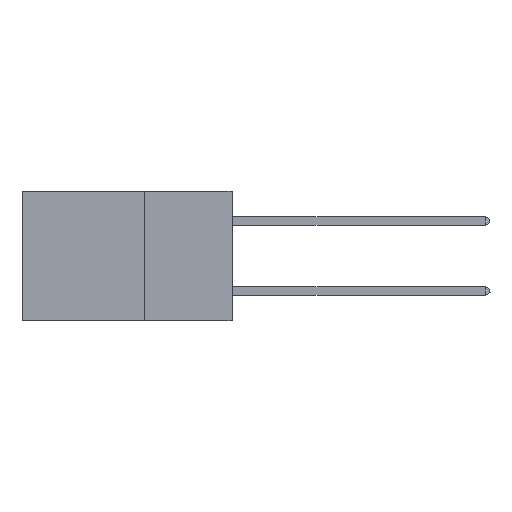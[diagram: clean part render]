
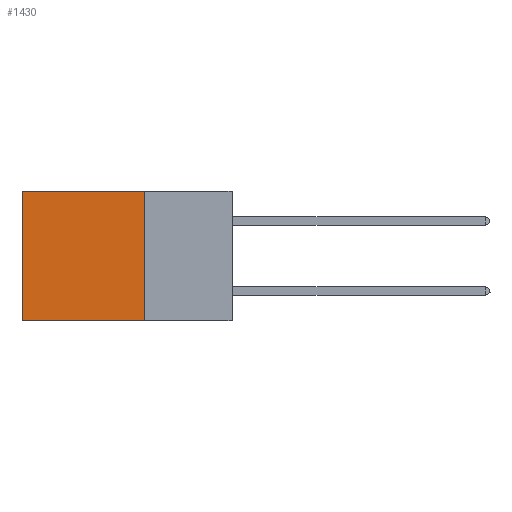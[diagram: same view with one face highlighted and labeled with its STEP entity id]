
A CAD part, left-side view. The second image highlights one B-rep face of the part: STEP entity #1430.
In plain terms, the highlighted planar face has unit normal (-1, 0, 0).
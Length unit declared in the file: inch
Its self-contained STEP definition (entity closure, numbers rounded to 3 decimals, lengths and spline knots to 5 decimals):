
#1430 = ADVANCED_FACE ( 'NONE', ( #26411 ), #11141, .F. ) ;
#1748 = VECTOR ( 'NONE', #10287, 39.37008 ) ;
#2034 = CARTESIAN_POINT ( 'NONE',  ( 0.2875, 0.25, 0. ) ) ;
#2132 = EDGE_CURVE ( 'NONE', #10776, #23455, #20278, .T. ) ;
#3590 = CARTESIAN_POINT ( 'NONE',  ( 0.2875, 0.25, -0.37 ) ) ;
#4003 = CARTESIAN_POINT ( 'NONE',  ( 0.2875, 0.6, -0.37 ) ) ;
#6883 = VERTEX_POINT ( 'NONE', #15807 ) ;
#7451 = CARTESIAN_POINT ( 'NONE',  ( 0.2875, 0.6, 0. ) ) ;
#9181 = LINE ( 'NONE', #15652, #20082 ) ;
#9241 = CARTESIAN_POINT ( 'NONE',  ( 0.2875, 0.25, 0. ) ) ;
#10201 = ORIENTED_EDGE ( 'NONE', *, *, #2132, .T. ) ;
#10287 = DIRECTION ( 'NONE',  ( 0., 1., 0. ) ) ;
#10776 = VERTEX_POINT ( 'NONE', #7451 ) ;
#11141 = PLANE ( 'NONE',  #11647 ) ;
#11647 = AXIS2_PLACEMENT_3D ( 'NONE', #9241, #23399, #19271 ) ;
#14461 = EDGE_CURVE ( 'NONE', #6883, #18330, #24735, .T. ) ;
#15525 = CARTESIAN_POINT ( 'NONE',  ( 0.2875, 0.25, -0.37 ) ) ;
#15572 = DIRECTION ( 'NONE',  ( 0., 1., 0. ) ) ;
#15652 = CARTESIAN_POINT ( 'NONE',  ( 0.2875, 0.25, 0. ) ) ;
#15807 = CARTESIAN_POINT ( 'NONE',  ( 0.2875, 0.25, 0. ) ) ;
#15849 = ORIENTED_EDGE ( 'NONE', *, *, #14461, .F. ) ;
#18330 = VERTEX_POINT ( 'NONE', #3590 ) ;
#18477 = ORIENTED_EDGE ( 'NONE', *, *, #25209, .F. ) ;
#19271 = DIRECTION ( 'NONE',  ( 0., 0., -1. ) ) ;
#19304 = LINE ( 'NONE', #15525, #1748 ) ;
#20082 = VECTOR ( 'NONE', #15572, 39.37008 ) ;
#20180 = DIRECTION ( 'NONE',  ( 0., 0., -1. ) ) ;
#20278 = LINE ( 'NONE', #25942, #24786 ) ;
#22277 = EDGE_CURVE ( 'NONE', #6883, #10776, #9181, .T. ) ;
#22656 = EDGE_LOOP ( 'NONE', ( #10201, #18477, #15849, #24704 ) ) ;
#22819 = VECTOR ( 'NONE', #20180, 39.37008 ) ;
#23399 = DIRECTION ( 'NONE',  ( 1., 0., 0. ) ) ;
#23455 = VERTEX_POINT ( 'NONE', #4003 ) ;
#23784 = DIRECTION ( 'NONE',  ( 0., 0., -1. ) ) ;
#24704 = ORIENTED_EDGE ( 'NONE', *, *, #22277, .T. ) ;
#24735 = LINE ( 'NONE', #2034, #22819 ) ;
#24786 = VECTOR ( 'NONE', #23784, 39.37008 ) ;
#25209 = EDGE_CURVE ( 'NONE', #18330, #23455, #19304, .T. ) ;
#25942 = CARTESIAN_POINT ( 'NONE',  ( 0.2875, 0.6, 0. ) ) ;
#26411 = FACE_OUTER_BOUND ( 'NONE', #22656, .T. ) ;
